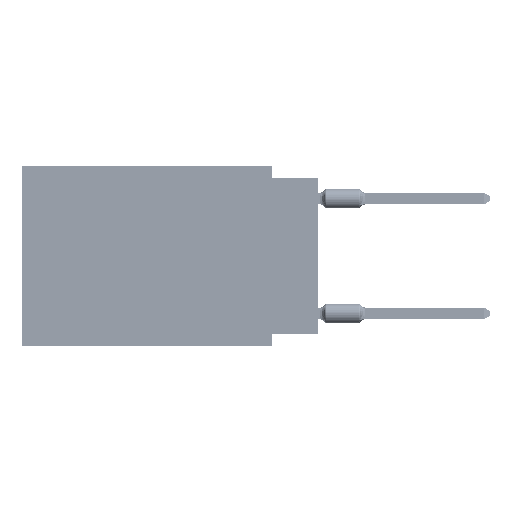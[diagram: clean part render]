
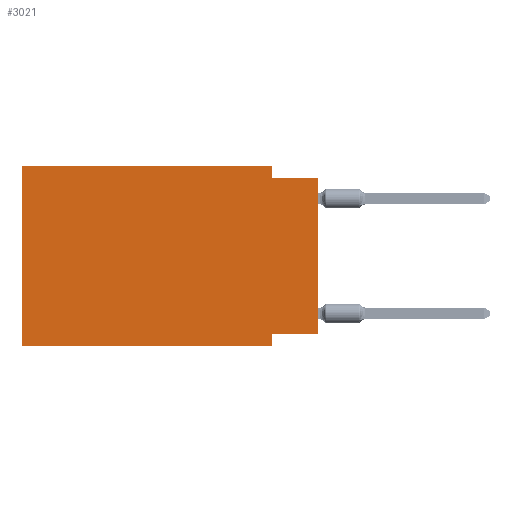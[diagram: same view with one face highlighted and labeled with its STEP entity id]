
A CAD part, left-side view. The second image highlights one B-rep face of the part: STEP entity #3021.
In plain terms, the highlighted planar face has unit normal (-1, 0, 0).
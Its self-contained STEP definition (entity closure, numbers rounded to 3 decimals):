
#1420 = CARTESIAN_POINT ( 'NONE',  ( 0., 0., 0. ) ) ;
#3021 = ADVANCED_FACE ( 'NONE', ( #10782 ), #11166, .F. ) ;
#5725 = LINE ( 'NONE', #66075, #42626 ) ;
#6757 = DIRECTION ( 'NONE',  ( 0., 1., 0. ) ) ;
#7330 = VECTOR ( 'NONE', #43111, 1000. ) ;
#8046 = DIRECTION ( 'NONE',  ( 0., 0., 1. ) ) ;
#8919 = VECTOR ( 'NONE', #54773, 1000. ) ;
#9387 = CARTESIAN_POINT ( 'NONE',  ( 0., 16.383, 0. ) ) ;
#10465 = VERTEX_POINT ( 'NONE', #70959 ) ;
#10782 = FACE_OUTER_BOUND ( 'NONE', #62855, .T. ) ;
#11166 = PLANE ( 'NONE',  #54299 ) ;
#11500 = EDGE_CURVE ( 'NONE', #29968, #57272, #5725, .T. ) ;
#12249 = LINE ( 'NONE', #42460, #48086 ) ;
#12499 = CARTESIAN_POINT ( 'NONE',  ( 0., 2.54, -0.635 ) ) ;
#15858 = EDGE_CURVE ( 'NONE', #10465, #57272, #66843, .T. ) ;
#16505 = EDGE_CURVE ( 'NONE', #10465, #51277, #12249, .T. ) ;
#18164 = VERTEX_POINT ( 'NONE', #52682 ) ;
#18220 = DIRECTION ( 'NONE',  ( 0., -1., 0. ) ) ;
#19240 = CARTESIAN_POINT ( 'NONE',  ( 0., 16.383, -9.906 ) ) ;
#20450 = VERTEX_POINT ( 'NONE', #9387 ) ;
#21017 = CARTESIAN_POINT ( 'NONE',  ( 0., 2.54, -9.271 ) ) ;
#21747 = ORIENTED_EDGE ( 'NONE', *, *, #26246, .F. ) ;
#24282 = CARTESIAN_POINT ( 'NONE',  ( 0., 2.54, -9.906 ) ) ;
#26246 = EDGE_CURVE ( 'NONE', #51277, #63878, #60637, .T. ) ;
#27072 = VERTEX_POINT ( 'NONE', #19240 ) ;
#28805 = DIRECTION ( 'NONE',  ( 0., 0., -1. ) ) ;
#29968 = VERTEX_POINT ( 'NONE', #12499 ) ;
#30405 = VECTOR ( 'NONE', #76556, 1000. ) ;
#31334 = LINE ( 'NONE', #31715, #7330 ) ;
#31715 = CARTESIAN_POINT ( 'NONE',  ( 0., 16.383, 0. ) ) ;
#34713 = CARTESIAN_POINT ( 'NONE',  ( 0., 16.383, 0. ) ) ;
#35001 = DIRECTION ( 'NONE',  ( 0., -1., 0. ) ) ;
#35185 = DIRECTION ( 'NONE',  ( 0., 0., -1. ) ) ;
#37910 = VECTOR ( 'NONE', #8046, 1000. ) ;
#40887 = EDGE_CURVE ( 'NONE', #27072, #20450, #31334, .T. ) ;
#41460 = ORIENTED_EDGE ( 'NONE', *, *, #16505, .F. ) ;
#42460 = CARTESIAN_POINT ( 'NONE',  ( 0., 0., -9.271 ) ) ;
#42508 = ORIENTED_EDGE ( 'NONE', *, *, #11500, .F. ) ;
#42626 = VECTOR ( 'NONE', #18220, 1000. ) ;
#43111 = DIRECTION ( 'NONE',  ( 0., 0., 1. ) ) ;
#43178 = EDGE_CURVE ( 'NONE', #20450, #18164, #52680, .T. ) ;
#44475 = VECTOR ( 'NONE', #35001, 1000. ) ;
#46371 = CARTESIAN_POINT ( 'NONE',  ( 0., 16.383, -9.906 ) ) ;
#47234 = DIRECTION ( 'NONE',  ( 1., 0., 0. ) ) ;
#48086 = VECTOR ( 'NONE', #6757, 1000. ) ;
#48612 = ORIENTED_EDGE ( 'NONE', *, *, #76897, .T. ) ;
#49988 = ORIENTED_EDGE ( 'NONE', *, *, #40887, .F. ) ;
#50327 = VECTOR ( 'NONE', #35185, 1000. ) ;
#51277 = VERTEX_POINT ( 'NONE', #21017 ) ;
#52680 = LINE ( 'NONE', #64065, #30405 ) ;
#52682 = CARTESIAN_POINT ( 'NONE',  ( 0., 2.54, 0. ) ) ;
#52804 = CARTESIAN_POINT ( 'NONE',  ( 0., 2.54, 0. ) ) ;
#54299 = AXIS2_PLACEMENT_3D ( 'NONE', #34713, #47234, #28805 ) ;
#54385 = CARTESIAN_POINT ( 'NONE',  ( 0., 2.54, -9.906 ) ) ;
#54773 = DIRECTION ( 'NONE',  ( 0., 0., -1. ) ) ;
#57217 = CARTESIAN_POINT ( 'NONE',  ( 0., 0., -0.635 ) ) ;
#57272 = VERTEX_POINT ( 'NONE', #57217 ) ;
#60637 = LINE ( 'NONE', #54385, #8919 ) ;
#61692 = ORIENTED_EDGE ( 'NONE', *, *, #63060, .F. ) ;
#62855 = EDGE_LOOP ( 'NONE', ( #72361, #42508, #61692, #72271, #49988, #48612, #21747, #41460 ) ) ;
#63060 = EDGE_CURVE ( 'NONE', #18164, #29968, #70418, .T. ) ;
#63878 = VERTEX_POINT ( 'NONE', #24282 ) ;
#64065 = CARTESIAN_POINT ( 'NONE',  ( 0., 16.383, 0. ) ) ;
#64780 = LINE ( 'NONE', #46371, #44475 ) ;
#66075 = CARTESIAN_POINT ( 'NONE',  ( 0., 0., -0.635 ) ) ;
#66843 = LINE ( 'NONE', #1420, #37910 ) ;
#70418 = LINE ( 'NONE', #52804, #50327 ) ;
#70959 = CARTESIAN_POINT ( 'NONE',  ( 0., 0., -9.271 ) ) ;
#72271 = ORIENTED_EDGE ( 'NONE', *, *, #43178, .F. ) ;
#72361 = ORIENTED_EDGE ( 'NONE', *, *, #15858, .T. ) ;
#76556 = DIRECTION ( 'NONE',  ( 0., -1., 0. ) ) ;
#76897 = EDGE_CURVE ( 'NONE', #27072, #63878, #64780, .T. ) ;
